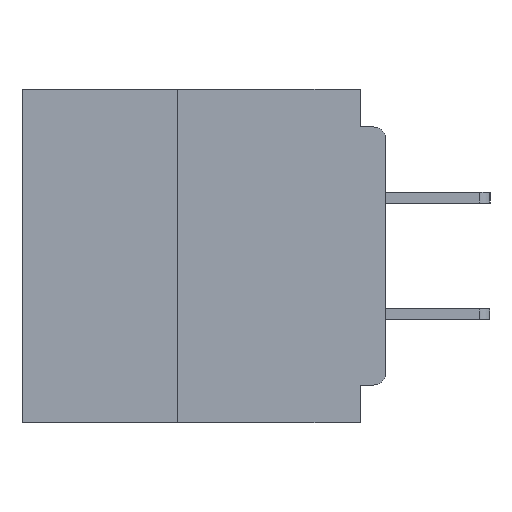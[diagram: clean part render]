
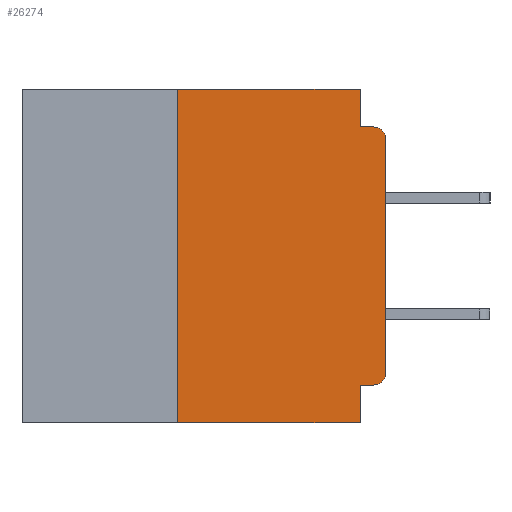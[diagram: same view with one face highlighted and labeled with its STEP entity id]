
A CAD part, left-side view. The second image highlights one B-rep face of the part: STEP entity #26274.
In plain terms, the highlighted planar face has unit normal (-1, 0, 0).
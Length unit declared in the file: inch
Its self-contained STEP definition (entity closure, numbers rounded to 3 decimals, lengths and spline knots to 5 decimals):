
#19 = VECTOR ( 'NONE', #26456, 39.37008 ) ;
#852 = AXIS2_PLACEMENT_3D ( 'NONE', #25863, #5616, #29264 ) ;
#1800 = LINE ( 'NONE', #11932, #24519 ) ;
#1916 = VECTOR ( 'NONE', #32697, 39.37008 ) ;
#2145 = EDGE_CURVE ( 'NONE', #16729, #29984, #9796, .T. ) ;
#2157 = VERTEX_POINT ( 'NONE', #22381 ) ;
#2258 = EDGE_CURVE ( 'NONE', #16392, #2157, #41490, .T. ) ;
#2602 = LINE ( 'NONE', #11254, #20602 ) ;
#2610 = ORIENTED_EDGE ( 'NONE', *, *, #14848, .T. ) ;
#5598 = VECTOR ( 'NONE', #23482, 39.37008 ) ;
#5616 = DIRECTION ( 'NONE',  ( -1., 0., 0. ) ) ;
#6671 = PLANE ( 'NONE',  #36867 ) ;
#8146 = DIRECTION ( 'NONE',  ( 0., -1., 0. ) ) ;
#8249 = ORIENTED_EDGE ( 'NONE', *, *, #10819, .T. ) ;
#9796 = LINE ( 'NONE', #26533, #1916 ) ;
#10031 = CARTESIAN_POINT ( 'NONE',  ( 0., 0.437, 0. ) ) ;
#10213 = CARTESIAN_POINT ( 'NONE',  ( 0., 0.031, -0.355 ) ) ;
#10819 = EDGE_CURVE ( 'NONE', #29984, #19865, #21726, .T. ) ;
#11037 = CARTESIAN_POINT ( 'NONE',  ( 0., 0.015, -0.34 ) ) ;
#11254 = CARTESIAN_POINT ( 'NONE',  ( 0., 0.031, 0. ) ) ;
#11932 = CARTESIAN_POINT ( 'NONE',  ( 0., 0.437, 0. ) ) ;
#11987 = CARTESIAN_POINT ( 'NONE',  ( 0., 0., -0.06 ) ) ;
#12616 = EDGE_CURVE ( 'NONE', #17226, #39894, #20041, .T. ) ;
#13067 = ORIENTED_EDGE ( 'NONE', *, *, #2145, .T. ) ;
#13432 = DIRECTION ( 'NONE',  ( 1., 0., 0. ) ) ;
#13988 = ORIENTED_EDGE ( 'NONE', *, *, #40088, .F. ) ;
#14455 = DIRECTION ( 'NONE',  ( 0., 0., -1. ) ) ;
#14674 = DIRECTION ( 'NONE',  ( 0., 0., -1. ) ) ;
#14848 = EDGE_CURVE ( 'NONE', #16392, #29419, #21948, .T. ) ;
#14961 = CARTESIAN_POINT ( 'NONE',  ( 0., 0., -0.34 ) ) ;
#15250 = LINE ( 'NONE', #34176, #25302 ) ;
#15371 = DIRECTION ( 'NONE',  ( 0., -1., 0. ) ) ;
#15441 = EDGE_CURVE ( 'NONE', #2157, #35982, #1800, .T. ) ;
#16392 = VERTEX_POINT ( 'NONE', #20477 ) ;
#16435 = CARTESIAN_POINT ( 'NONE',  ( 0., 0., -0.355 ) ) ;
#16729 = VERTEX_POINT ( 'NONE', #14961 ) ;
#16748 = CARTESIAN_POINT ( 'NONE',  ( 0., 0.015, -0.045 ) ) ;
#17226 = VERTEX_POINT ( 'NONE', #21582 ) ;
#17268 = ORIENTED_EDGE ( 'NONE', *, *, #36504, .T. ) ;
#17395 = ORIENTED_EDGE ( 'NONE', *, *, #27649, .F. ) ;
#18504 = CARTESIAN_POINT ( 'NONE',  ( 0., 0.031, 0. ) ) ;
#18655 = CARTESIAN_POINT ( 'NONE',  ( 0., 0.031, -0.045 ) ) ;
#18976 = VECTOR ( 'NONE', #19848, 39.37008 ) ;
#19848 = DIRECTION ( 'NONE',  ( 0., 1., 0. ) ) ;
#19865 = VERTEX_POINT ( 'NONE', #16748 ) ;
#20041 = LINE ( 'NONE', #16435, #18976 ) ;
#20477 = CARTESIAN_POINT ( 'NONE',  ( 0., 0.25, -0.4 ) ) ;
#20602 = VECTOR ( 'NONE', #14674, 39.37008 ) ;
#21178 = ORIENTED_EDGE ( 'NONE', *, *, #12616, .F. ) ;
#21582 = CARTESIAN_POINT ( 'NONE',  ( 0., 0.015, -0.355 ) ) ;
#21726 = CIRCLE ( 'NONE', #852, 0.015 ) ;
#21948 = LINE ( 'NONE', #25033, #38844 ) ;
#22381 = CARTESIAN_POINT ( 'NONE',  ( 0., 0.25, 0. ) ) ;
#22576 = CARTESIAN_POINT ( 'NONE',  ( 0., 0.031, -0.4 ) ) ;
#23054 = CARTESIAN_POINT ( 'NONE',  ( 0., 0., -0.045 ) ) ;
#23482 = DIRECTION ( 'NONE',  ( 0., 0., 1. ) ) ;
#24062 = EDGE_LOOP ( 'NONE', ( #13067, #8249, #32267, #13988, #35101, #39451, #2610, #17395, #21178, #17268 ) ) ;
#24519 = VECTOR ( 'NONE', #15371, 39.37008 ) ;
#25033 = CARTESIAN_POINT ( 'NONE',  ( 0., 0.437, -0.4 ) ) ;
#25302 = VECTOR ( 'NONE', #37577, 39.37008 ) ;
#25863 = CARTESIAN_POINT ( 'NONE',  ( 0., 0.015, -0.06 ) ) ;
#26274 = ADVANCED_FACE ( 'NONE', ( #43290 ), #6671, .F. ) ;
#26456 = DIRECTION ( 'NONE',  ( 0., -1., 0. ) ) ;
#26533 = CARTESIAN_POINT ( 'NONE',  ( 0., 0., 0. ) ) ;
#26987 = LINE ( 'NONE', #23054, #19 ) ;
#27649 = EDGE_CURVE ( 'NONE', #39894, #29419, #15250, .T. ) ;
#29264 = DIRECTION ( 'NONE',  ( 0., 0., -1. ) ) ;
#29419 = VERTEX_POINT ( 'NONE', #22576 ) ;
#29984 = VERTEX_POINT ( 'NONE', #11987 ) ;
#32267 = ORIENTED_EDGE ( 'NONE', *, *, #42854, .F. ) ;
#32697 = DIRECTION ( 'NONE',  ( 0., 0., 1. ) ) ;
#34141 = CIRCLE ( 'NONE', #39724, 0.015 ) ;
#34149 = VERTEX_POINT ( 'NONE', #18655 ) ;
#34176 = CARTESIAN_POINT ( 'NONE',  ( 0., 0.031, -0.4 ) ) ;
#34699 = DIRECTION ( 'NONE',  ( -1., 0., 0. ) ) ;
#35101 = ORIENTED_EDGE ( 'NONE', *, *, #15441, .F. ) ;
#35982 = VERTEX_POINT ( 'NONE', #18504 ) ;
#36504 = EDGE_CURVE ( 'NONE', #17226, #16729, #34141, .T. ) ;
#36867 = AXIS2_PLACEMENT_3D ( 'NONE', #10031, #13432, #37120 ) ;
#37120 = DIRECTION ( 'NONE',  ( 0., 0., -1. ) ) ;
#37577 = DIRECTION ( 'NONE',  ( 0., 0., -1. ) ) ;
#38844 = VECTOR ( 'NONE', #8146, 39.37008 ) ;
#39451 = ORIENTED_EDGE ( 'NONE', *, *, #2258, .F. ) ;
#39724 = AXIS2_PLACEMENT_3D ( 'NONE', #11037, #34699, #14455 ) ;
#39894 = VERTEX_POINT ( 'NONE', #10213 ) ;
#40088 = EDGE_CURVE ( 'NONE', #35982, #34149, #2602, .T. ) ;
#41490 = LINE ( 'NONE', #42421, #5598 ) ;
#42421 = CARTESIAN_POINT ( 'NONE',  ( 0., 0.25, -0.4 ) ) ;
#42854 = EDGE_CURVE ( 'NONE', #34149, #19865, #26987, .T. ) ;
#43290 = FACE_OUTER_BOUND ( 'NONE', #24062, .T. ) ;
